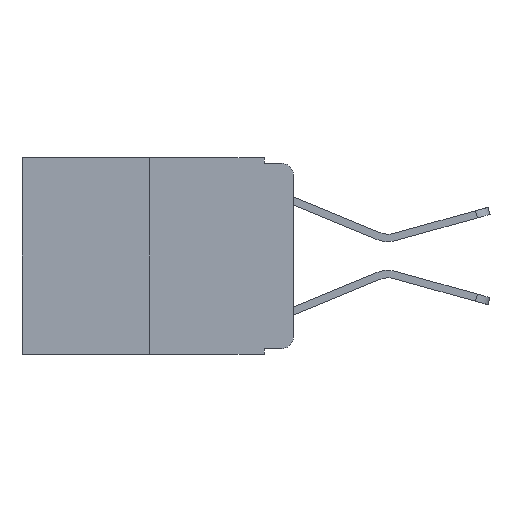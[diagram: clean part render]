
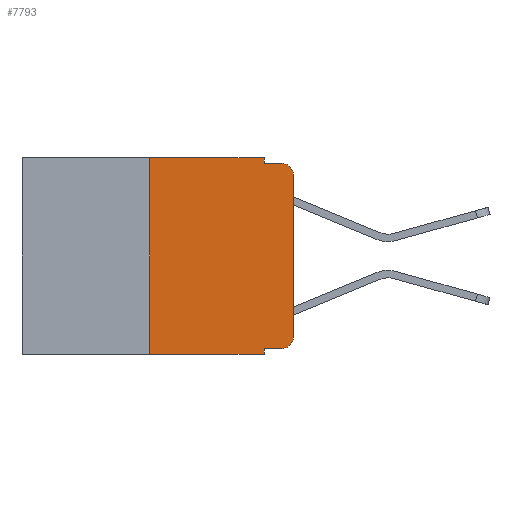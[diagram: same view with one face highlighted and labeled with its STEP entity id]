
A CAD part, left-side view. The second image highlights one B-rep face of the part: STEP entity #7793.
In plain terms, the highlighted planar face has unit normal (-1, 0, 0).
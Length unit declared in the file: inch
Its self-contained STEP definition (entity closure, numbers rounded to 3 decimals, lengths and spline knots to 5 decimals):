
#401 = CARTESIAN_POINT ( 'NONE',  ( 0., 0.051, -0.01 ) ) ;
#819 = VERTEX_POINT ( 'NONE', #7274 ) ;
#878 = DIRECTION ( 'NONE',  ( 0., 0., -1. ) ) ;
#1439 = EDGE_CURVE ( 'NONE', #13124, #1524, #17635, .T. ) ;
#1512 = VECTOR ( 'NONE', #25684, 39.37008 ) ;
#1524 = VERTEX_POINT ( 'NONE', #12840 ) ;
#1585 = LINE ( 'NONE', #3697, #22464 ) ;
#1678 = DIRECTION ( 'NONE',  ( 1., 0., 0. ) ) ;
#1863 = CARTESIAN_POINT ( 'NONE',  ( 0., 0.051, -0.01 ) ) ;
#1941 = CARTESIAN_POINT ( 'NONE',  ( 0., 0.473, 0. ) ) ;
#3092 = VECTOR ( 'NONE', #10397, 39.37008 ) ;
#3386 = LINE ( 'NONE', #5619, #24805 ) ;
#3605 = CARTESIAN_POINT ( 'NONE',  ( 0., 0., -0.03 ) ) ;
#3697 = CARTESIAN_POINT ( 'NONE',  ( 0., 0.051, -0.333 ) ) ;
#3952 = EDGE_CURVE ( 'NONE', #25465, #18366, #13808, .T. ) ;
#4017 = VERTEX_POINT ( 'NONE', #3605 ) ;
#4178 = DIRECTION ( 'NONE',  ( 0., 0., -1. ) ) ;
#5484 = DIRECTION ( 'NONE',  ( 0., -1., 0. ) ) ;
#5619 = CARTESIAN_POINT ( 'NONE',  ( 0., 0.473, 0. ) ) ;
#5693 = VECTOR ( 'NONE', #878, 39.37008 ) ;
#5870 = VECTOR ( 'NONE', #16788, 39.37008 ) ;
#5945 = DIRECTION ( 'NONE',  ( 0., 0., -1. ) ) ;
#6486 = EDGE_LOOP ( 'NONE', ( #12587, #25067, #12051, #13120, #22325, #12961, #8519, #15871, #12081, #20249 ) ) ;
#7096 = CARTESIAN_POINT ( 'NONE',  ( 0., 0., -0.313 ) ) ;
#7274 = CARTESIAN_POINT ( 'NONE',  ( 0., 0.051, -0.343 ) ) ;
#7527 = DIRECTION ( 'NONE',  ( -1., 0., 0. ) ) ;
#7793 = ADVANCED_FACE ( 'NONE', ( #23781 ), #18100, .F. ) ;
#8115 = AXIS2_PLACEMENT_3D ( 'NONE', #1941, #1678, #4178 ) ;
#8519 = ORIENTED_EDGE ( 'NONE', *, *, #14878, .T. ) ;
#8553 = LINE ( 'NONE', #11976, #3092 ) ;
#8600 = LINE ( 'NONE', #18489, #24475 ) ;
#8879 = CARTESIAN_POINT ( 'NONE',  ( 0., 0.051, 0. ) ) ;
#9139 = EDGE_CURVE ( 'NONE', #17959, #25465, #1585, .T. ) ;
#10397 = DIRECTION ( 'NONE',  ( 0., 0., -1. ) ) ;
#10436 = CARTESIAN_POINT ( 'NONE',  ( 0., 0.02, -0.03 ) ) ;
#10951 = DIRECTION ( 'NONE',  ( 0., 0., -1. ) ) ;
#11079 = EDGE_CURVE ( 'NONE', #18366, #4017, #11343, .T. ) ;
#11343 = LINE ( 'NONE', #25567, #1512 ) ;
#11587 = VECTOR ( 'NONE', #13679, 39.37008 ) ;
#11976 = CARTESIAN_POINT ( 'NONE',  ( 0., 0.051, 0. ) ) ;
#12051 = ORIENTED_EDGE ( 'NONE', *, *, #1439, .F. ) ;
#12081 = ORIENTED_EDGE ( 'NONE', *, *, #9139, .T. ) ;
#12135 = VERTEX_POINT ( 'NONE', #25629 ) ;
#12185 = CARTESIAN_POINT ( 'NONE',  ( 0., 0.25, 0. ) ) ;
#12410 = VERTEX_POINT ( 'NONE', #17255 ) ;
#12587 = ORIENTED_EDGE ( 'NONE', *, *, #11079, .T. ) ;
#12840 = CARTESIAN_POINT ( 'NONE',  ( 0., 0.02, -0.01 ) ) ;
#12961 = ORIENTED_EDGE ( 'NONE', *, *, #23118, .F. ) ;
#13120 = ORIENTED_EDGE ( 'NONE', *, *, #22774, .F. ) ;
#13124 = VERTEX_POINT ( 'NONE', #401 ) ;
#13679 = DIRECTION ( 'NONE',  ( 0., -1., 0. ) ) ;
#13808 = CIRCLE ( 'NONE', #15912, 0.02 ) ;
#14560 = CARTESIAN_POINT ( 'NONE',  ( 0., 0.473, -0.343 ) ) ;
#14769 = DIRECTION ( 'NONE',  ( 0., 0., 1. ) ) ;
#14794 = VERTEX_POINT ( 'NONE', #12185 ) ;
#14878 = EDGE_CURVE ( 'NONE', #12135, #819, #14946, .T. ) ;
#14946 = LINE ( 'NONE', #14560, #5870 ) ;
#15871 = ORIENTED_EDGE ( 'NONE', *, *, #20487, .F. ) ;
#15912 = AXIS2_PLACEMENT_3D ( 'NONE', #25570, #7527, #5945 ) ;
#15935 = EDGE_CURVE ( 'NONE', #14794, #12410, #3386, .T. ) ;
#16477 = AXIS2_PLACEMENT_3D ( 'NONE', #10436, #25053, #10951 ) ;
#16647 = LINE ( 'NONE', #8879, #5693 ) ;
#16788 = DIRECTION ( 'NONE',  ( 0., -1., 0. ) ) ;
#17255 = CARTESIAN_POINT ( 'NONE',  ( 0., 0.051, 0. ) ) ;
#17625 = DIRECTION ( 'NONE',  ( 0., -1., 0. ) ) ;
#17635 = LINE ( 'NONE', #1863, #11587 ) ;
#17959 = VERTEX_POINT ( 'NONE', #18474 ) ;
#18100 = PLANE ( 'NONE',  #8115 ) ;
#18366 = VERTEX_POINT ( 'NONE', #7096 ) ;
#18474 = CARTESIAN_POINT ( 'NONE',  ( 0., 0.051, -0.333 ) ) ;
#18489 = CARTESIAN_POINT ( 'NONE',  ( 0., 0.25, 0. ) ) ;
#18563 = CARTESIAN_POINT ( 'NONE',  ( 0., 0.02, -0.333 ) ) ;
#20249 = ORIENTED_EDGE ( 'NONE', *, *, #3952, .T. ) ;
#20487 = EDGE_CURVE ( 'NONE', #17959, #819, #8553, .T. ) ;
#22325 = ORIENTED_EDGE ( 'NONE', *, *, #15935, .F. ) ;
#22464 = VECTOR ( 'NONE', #17625, 39.37008 ) ;
#22774 = EDGE_CURVE ( 'NONE', #12410, #13124, #16647, .T. ) ;
#23118 = EDGE_CURVE ( 'NONE', #12135, #14794, #8600, .T. ) ;
#23183 = EDGE_CURVE ( 'NONE', #4017, #1524, #25736, .T. ) ;
#23781 = FACE_OUTER_BOUND ( 'NONE', #6486, .T. ) ;
#24475 = VECTOR ( 'NONE', #14769, 39.37008 ) ;
#24805 = VECTOR ( 'NONE', #5484, 39.37008 ) ;
#25053 = DIRECTION ( 'NONE',  ( -1., 0., 0. ) ) ;
#25067 = ORIENTED_EDGE ( 'NONE', *, *, #23183, .T. ) ;
#25465 = VERTEX_POINT ( 'NONE', #18563 ) ;
#25567 = CARTESIAN_POINT ( 'NONE',  ( 0., 0., 0. ) ) ;
#25570 = CARTESIAN_POINT ( 'NONE',  ( 0., 0.02, -0.313 ) ) ;
#25629 = CARTESIAN_POINT ( 'NONE',  ( 0., 0.25, -0.343 ) ) ;
#25684 = DIRECTION ( 'NONE',  ( 0., 0., 1. ) ) ;
#25736 = CIRCLE ( 'NONE', #16477, 0.02 ) ;
